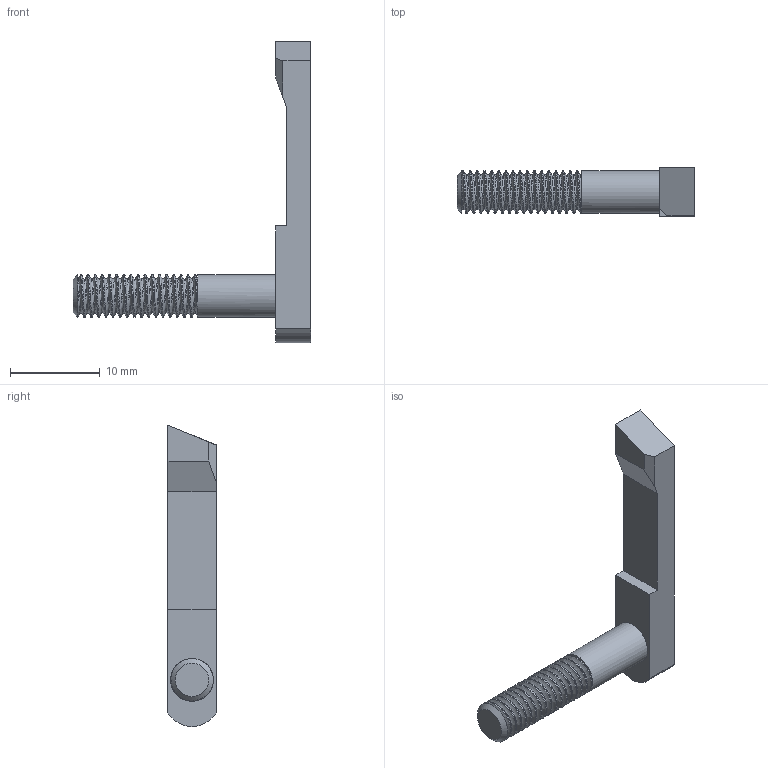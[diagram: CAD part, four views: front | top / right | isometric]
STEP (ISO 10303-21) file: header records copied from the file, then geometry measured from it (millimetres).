
FILE_DESCRIPTION(/* description */ (''),/* implementation_level */ '2;1');
FILE_NAME(/* name */ 'AR Magazine Catch modified.step',/* time_stamp */ '2024-01-16T15:56:02-05:00',/* author */ (''),/* organization */ (''),/* preprocessor_version */ 'ST-DEVELOPER v20',/* originating_system */ 'Autodesk Translation Framework v12.14.0.127',/* authorisation */ '');
FILE_SCHEMA (('AUTOMOTIVE_DESIGN { 1 0 10303 214 3 1 1 }'));
Length unit declared in the file: inch
Products named in the file (1): AR Magazine Catch
Bounding box: 26.39 x 5.33 x 33.46 mm (x, y, z)
Volume: 917.2 mm3; surface area: 1028.8 mm2
Topology: 1 solids, 1 shells, 53 faces, 148 edges, 98 vertices
Faces by surface type: cylinder 37, plane 13, bspline 2, cone 1
Full cylindrical faces by diameter (mm): 3.858 x6, 4.727 x12
Entity records: 3672 total; most frequent: CARTESIAN_POINT 2415, ORIENTED_EDGE 296, DIRECTION 189, EDGE_CURVE 148, VERTEX_POINT 98, B_SPLINE_CURVE_WITH_KNOTS 75, AXIS2_PLACEMENT_3D 64, LINE 61
